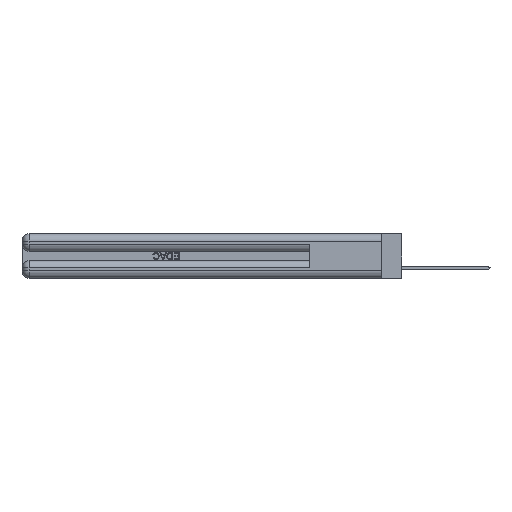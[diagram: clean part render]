
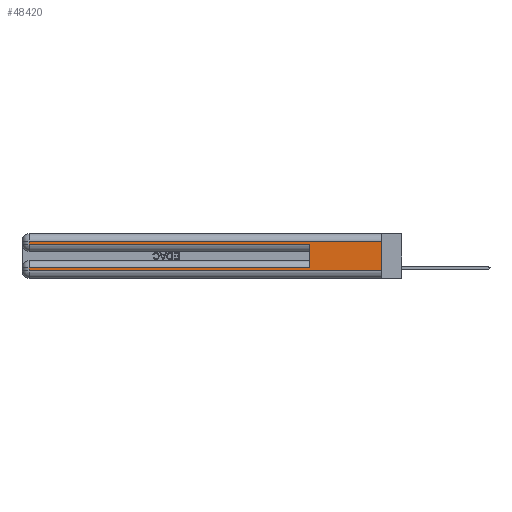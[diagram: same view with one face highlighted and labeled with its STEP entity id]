
A CAD part, left-side view. The second image highlights one B-rep face of the part: STEP entity #48420.
In plain terms, the highlighted planar face has unit normal (-1, 0, 0).
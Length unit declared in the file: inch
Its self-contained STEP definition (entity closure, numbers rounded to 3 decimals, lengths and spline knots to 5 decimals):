
#293 = ORIENTED_EDGE ( 'NONE', *, *, #46663, .F. ) ;
#1389 = AXIS2_PLACEMENT_3D ( 'NONE', #49268, #14196, #18214 ) ;
#2086 = CARTESIAN_POINT ( 'NONE',  ( 0., 2.94, 0.06 ) ) ;
#3150 = EDGE_CURVE ( 'NONE', #28957, #38759, #40542, .T. ) ;
#3259 = VERTEX_POINT ( 'NONE', #23661 ) ;
#4036 = VECTOR ( 'NONE', #36335, 39.37008 ) ;
#6417 = CARTESIAN_POINT ( 'NONE',  ( 0., 0.6, 0.085 ) ) ;
#6682 = EDGE_CURVE ( 'NONE', #7663, #31832, #43162, .T. ) ;
#7163 = DIRECTION ( 'NONE',  ( 0., 1., 0. ) ) ;
#7663 = VERTEX_POINT ( 'NONE', #6417 ) ;
#7702 = LINE ( 'NONE', #47679, #4036 ) ;
#7977 = EDGE_CURVE ( 'NONE', #19202, #49076, #16485, .T. ) ;
#8442 = EDGE_CURVE ( 'NONE', #46799, #3259, #25522, .T. ) ;
#8466 = ORIENTED_EDGE ( 'NONE', *, *, #6682, .T. ) ;
#8771 = DIRECTION ( 'NONE',  ( 0., -1., 0. ) ) ;
#10329 = PLANE ( 'NONE',  #1389 ) ;
#11692 = LINE ( 'NONE', #37908, #35235 ) ;
#14038 = ORIENTED_EDGE ( 'NONE', *, *, #3150, .T. ) ;
#14196 = DIRECTION ( 'NONE',  ( 1., 0., 0. ) ) ;
#15375 = CARTESIAN_POINT ( 'NONE',  ( 0., 0., 0.085 ) ) ;
#15766 = EDGE_CURVE ( 'NONE', #7663, #49076, #7702, .T. ) ;
#16485 = LINE ( 'NONE', #21161, #46034 ) ;
#17441 = ORIENTED_EDGE ( 'NONE', *, *, #37211, .T. ) ;
#18214 = DIRECTION ( 'NONE',  ( 0., 0., -1. ) ) ;
#18499 = DIRECTION ( 'NONE',  ( 0., 0., -1. ) ) ;
#18634 = CARTESIAN_POINT ( 'NONE',  ( 0., 0.6, 0.285 ) ) ;
#19102 = FACE_OUTER_BOUND ( 'NONE', #26011, .T. ) ;
#19173 = CARTESIAN_POINT ( 'NONE',  ( 0., 0., 0.06 ) ) ;
#19202 = VERTEX_POINT ( 'NONE', #37263 ) ;
#20636 = DIRECTION ( 'NONE',  ( 0., 0., -1. ) ) ;
#21161 = CARTESIAN_POINT ( 'NONE',  ( 0., 0., 0.285 ) ) ;
#21819 = VECTOR ( 'NONE', #20636, 39.37008 ) ;
#23484 = CARTESIAN_POINT ( 'NONE',  ( 0., 0., 0.31 ) ) ;
#23661 = CARTESIAN_POINT ( 'NONE',  ( 0., 2.94, 0.31 ) ) ;
#25522 = LINE ( 'NONE', #37879, #48957 ) ;
#26011 = EDGE_LOOP ( 'NONE', ( #293, #30023, #43719, #31114, #42061, #8466, #17441, #14038 ) ) ;
#27918 = CARTESIAN_POINT ( 'NONE',  ( 0., 0., 0.06 ) ) ;
#28957 = VERTEX_POINT ( 'NONE', #2086 ) ;
#30023 = ORIENTED_EDGE ( 'NONE', *, *, #8442, .T. ) ;
#30809 = CARTESIAN_POINT ( 'NONE',  ( 0., 2.94, 0.085 ) ) ;
#31114 = ORIENTED_EDGE ( 'NONE', *, *, #7977, .T. ) ;
#31832 = VERTEX_POINT ( 'NONE', #30809 ) ;
#32973 = VECTOR ( 'NONE', #7163, 39.37008 ) ;
#34409 = LINE ( 'NONE', #34594, #42205 ) ;
#34594 = CARTESIAN_POINT ( 'NONE',  ( 0., 0., 0.37 ) ) ;
#35235 = VECTOR ( 'NONE', #18499, 39.37008 ) ;
#36335 = DIRECTION ( 'NONE',  ( 0., 0., 1. ) ) ;
#37211 = EDGE_CURVE ( 'NONE', #31832, #28957, #11692, .T. ) ;
#37263 = CARTESIAN_POINT ( 'NONE',  ( 0., 2.94, 0.285 ) ) ;
#37879 = CARTESIAN_POINT ( 'NONE',  ( 0., 0., 0.31 ) ) ;
#37908 = CARTESIAN_POINT ( 'NONE',  ( 0., 2.94, 0.37 ) ) ;
#38288 = DIRECTION ( 'NONE',  ( 0., 0., -1. ) ) ;
#38759 = VERTEX_POINT ( 'NONE', #19173 ) ;
#39862 = LINE ( 'NONE', #40746, #21819 ) ;
#40542 = LINE ( 'NONE', #27918, #49510 ) ;
#40746 = CARTESIAN_POINT ( 'NONE',  ( 0., 2.94, 0.37 ) ) ;
#42061 = ORIENTED_EDGE ( 'NONE', *, *, #15766, .F. ) ;
#42205 = VECTOR ( 'NONE', #38288, 39.37008 ) ;
#43162 = LINE ( 'NONE', #15375, #32973 ) ;
#43719 = ORIENTED_EDGE ( 'NONE', *, *, #45436, .T. ) ;
#45410 = DIRECTION ( 'NONE',  ( 0., 1., 0. ) ) ;
#45436 = EDGE_CURVE ( 'NONE', #3259, #19202, #39862, .T. ) ;
#46034 = VECTOR ( 'NONE', #48570, 39.37008 ) ;
#46663 = EDGE_CURVE ( 'NONE', #46799, #38759, #34409, .T. ) ;
#46799 = VERTEX_POINT ( 'NONE', #23484 ) ;
#47679 = CARTESIAN_POINT ( 'NONE',  ( 0., 0.6, 0.145 ) ) ;
#48420 = ADVANCED_FACE ( 'NONE', ( #19102 ), #10329, .F. ) ;
#48570 = DIRECTION ( 'NONE',  ( 0., -1., 0. ) ) ;
#48957 = VECTOR ( 'NONE', #45410, 39.37008 ) ;
#49076 = VERTEX_POINT ( 'NONE', #18634 ) ;
#49268 = CARTESIAN_POINT ( 'NONE',  ( 0., 0., 0.37 ) ) ;
#49510 = VECTOR ( 'NONE', #8771, 39.37008 ) ;
